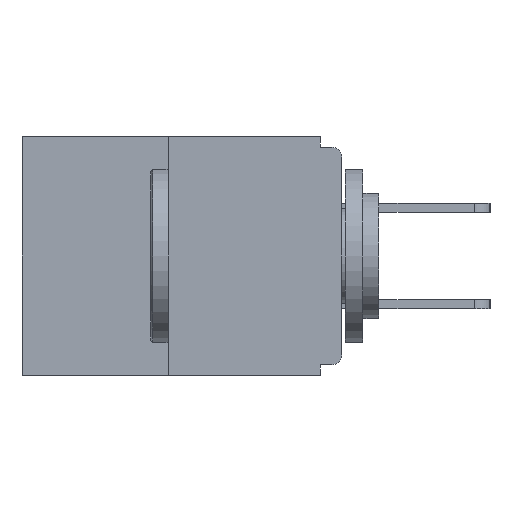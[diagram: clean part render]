
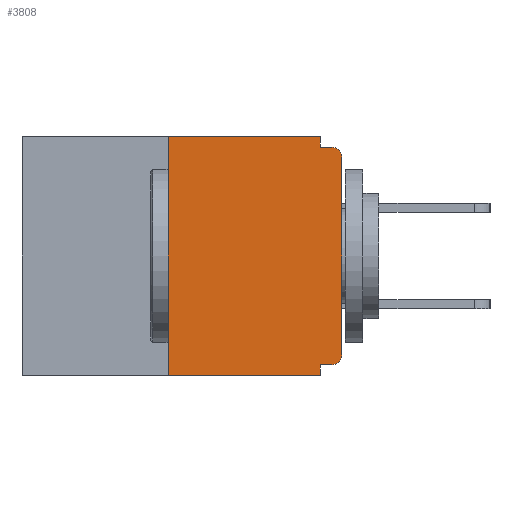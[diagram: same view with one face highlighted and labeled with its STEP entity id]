
A CAD part, left-side view. The second image highlights one B-rep face of the part: STEP entity #3808.
In plain terms, the highlighted planar face has unit normal (-1, 0, 0).
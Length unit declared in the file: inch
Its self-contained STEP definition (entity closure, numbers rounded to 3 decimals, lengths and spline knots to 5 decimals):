
#72 = LINE ( 'NONE', #8200, #8737 ) ;
#194 = CARTESIAN_POINT ( 'NONE',  ( 0., 0.031, -0.328 ) ) ;
#492 = LINE ( 'NONE', #3916, #2522 ) ;
#623 = LINE ( 'NONE', #11089, #8956 ) ;
#651 = ORIENTED_EDGE ( 'NONE', *, *, #4061, .T. ) ;
#663 = CARTESIAN_POINT ( 'NONE',  ( 0., 0.015, -0.328 ) ) ;
#784 = VECTOR ( 'NONE', #2452, 39.37008 ) ;
#804 = VERTEX_POINT ( 'NONE', #7273 ) ;
#844 = DIRECTION ( 'NONE',  ( -1., 0., 0. ) ) ;
#850 = DIRECTION ( 'NONE',  ( 0., 0., -1. ) ) ;
#1008 = AXIS2_PLACEMENT_3D ( 'NONE', #3945, #1870, #2927 ) ;
#1231 = EDGE_CURVE ( 'NONE', #7471, #804, #9520, .T. ) ;
#1250 = CARTESIAN_POINT ( 'NONE',  ( 0., 0.015, -0.015 ) ) ;
#1302 = ORIENTED_EDGE ( 'NONE', *, *, #5220, .F. ) ;
#1521 = EDGE_CURVE ( 'NONE', #3811, #3905, #72, .T. ) ;
#1755 = VERTEX_POINT ( 'NONE', #3054 ) ;
#1815 = CARTESIAN_POINT ( 'NONE',  ( 0., 0.031, -0.343 ) ) ;
#1870 = DIRECTION ( 'NONE',  ( -1., 0., 0. ) ) ;
#1968 = DIRECTION ( 'NONE',  ( 0., 0., -1. ) ) ;
#1997 = DIRECTION ( 'NONE',  ( 0., -1., 0. ) ) ;
#2021 = LINE ( 'NONE', #8371, #784 ) ;
#2122 = ORIENTED_EDGE ( 'NONE', *, *, #1521, .F. ) ;
#2430 = CARTESIAN_POINT ( 'NONE',  ( 0., 0.46, 0. ) ) ;
#2452 = DIRECTION ( 'NONE',  ( 0., 0., 1. ) ) ;
#2522 = VECTOR ( 'NONE', #11667, 39.37008 ) ;
#2750 = CARTESIAN_POINT ( 'NONE',  ( 0., 0.031, 0. ) ) ;
#2927 = DIRECTION ( 'NONE',  ( 0., 0., -1. ) ) ;
#2958 = LINE ( 'NONE', #2750, #9585 ) ;
#3054 = CARTESIAN_POINT ( 'NONE',  ( 0., 0.031, -0.015 ) ) ;
#3327 = DIRECTION ( 'NONE',  ( 0., 0., -1. ) ) ;
#3495 = PLANE ( 'NONE',  #10316 ) ;
#3754 = VERTEX_POINT ( 'NONE', #194 ) ;
#3802 = VERTEX_POINT ( 'NONE', #11382 ) ;
#3808 = ADVANCED_FACE ( 'NONE', ( #6833 ), #3495, .F. ) ;
#3811 = VERTEX_POINT ( 'NONE', #6304 ) ;
#3905 = VERTEX_POINT ( 'NONE', #7506 ) ;
#3916 = CARTESIAN_POINT ( 'NONE',  ( 0., 0., -0.328 ) ) ;
#3945 = CARTESIAN_POINT ( 'NONE',  ( 0., 0.015, -0.03 ) ) ;
#4061 = EDGE_CURVE ( 'NONE', #804, #8149, #8849, .T. ) ;
#4160 = EDGE_CURVE ( 'NONE', #7471, #3754, #492, .T. ) ;
#4607 = LINE ( 'NONE', #9887, #12474 ) ;
#4749 = ORIENTED_EDGE ( 'NONE', *, *, #4160, .F. ) ;
#4822 = DIRECTION ( 'NONE',  ( 0., 0., 1. ) ) ;
#5002 = EDGE_CURVE ( 'NONE', #10737, #3811, #2021, .T. ) ;
#5121 = ORIENTED_EDGE ( 'NONE', *, *, #11349, .F. ) ;
#5173 = ORIENTED_EDGE ( 'NONE', *, *, #10249, .F. ) ;
#5220 = EDGE_CURVE ( 'NONE', #3905, #1755, #2958, .T. ) ;
#5342 = ORIENTED_EDGE ( 'NONE', *, *, #7590, .T. ) ;
#5391 = EDGE_CURVE ( 'NONE', #10737, #3802, #623, .T. ) ;
#5588 = DIRECTION ( 'NONE',  ( 0., 0., -1. ) ) ;
#5977 = VECTOR ( 'NONE', #850, 39.37008 ) ;
#6135 = DIRECTION ( 'NONE',  ( 0., -1., 0. ) ) ;
#6304 = CARTESIAN_POINT ( 'NONE',  ( 0., 0.25, 0. ) ) ;
#6742 = LINE ( 'NONE', #1815, #5977 ) ;
#6798 = CARTESIAN_POINT ( 'NONE',  ( 0., 0.015, -0.313 ) ) ;
#6833 = FACE_OUTER_BOUND ( 'NONE', #10438, .T. ) ;
#7273 = CARTESIAN_POINT ( 'NONE',  ( 0., 0., -0.313 ) ) ;
#7323 = DIRECTION ( 'NONE',  ( 1., 0., 0. ) ) ;
#7471 = VERTEX_POINT ( 'NONE', #663 ) ;
#7506 = CARTESIAN_POINT ( 'NONE',  ( 0., 0.031, 0. ) ) ;
#7590 = EDGE_CURVE ( 'NONE', #8149, #12725, #12071, .T. ) ;
#8149 = VERTEX_POINT ( 'NONE', #10561 ) ;
#8200 = CARTESIAN_POINT ( 'NONE',  ( 0., 0.46, 0. ) ) ;
#8371 = CARTESIAN_POINT ( 'NONE',  ( 0., 0.25, 0. ) ) ;
#8687 = VECTOR ( 'NONE', #4822, 39.37008 ) ;
#8737 = VECTOR ( 'NONE', #10193, 39.37008 ) ;
#8849 = LINE ( 'NONE', #12632, #8687 ) ;
#8925 = ORIENTED_EDGE ( 'NONE', *, *, #5391, .T. ) ;
#8956 = VECTOR ( 'NONE', #6135, 39.37008 ) ;
#9520 = CIRCLE ( 'NONE', #9808, 0.015 ) ;
#9585 = VECTOR ( 'NONE', #5588, 39.37008 ) ;
#9717 = CARTESIAN_POINT ( 'NONE',  ( 0., 0.25, -0.343 ) ) ;
#9808 = AXIS2_PLACEMENT_3D ( 'NONE', #6798, #844, #1968 ) ;
#9887 = CARTESIAN_POINT ( 'NONE',  ( 0., 0., -0.015 ) ) ;
#10193 = DIRECTION ( 'NONE',  ( 0., -1., 0. ) ) ;
#10249 = EDGE_CURVE ( 'NONE', #1755, #12725, #4607, .T. ) ;
#10316 = AXIS2_PLACEMENT_3D ( 'NONE', #2430, #7323, #3327 ) ;
#10438 = EDGE_LOOP ( 'NONE', ( #2122, #11658, #8925, #5121, #4749, #11987, #651, #5342, #5173, #1302 ) ) ;
#10561 = CARTESIAN_POINT ( 'NONE',  ( 0., 0., -0.03 ) ) ;
#10737 = VERTEX_POINT ( 'NONE', #9717 ) ;
#11089 = CARTESIAN_POINT ( 'NONE',  ( 0., 0.46, -0.343 ) ) ;
#11349 = EDGE_CURVE ( 'NONE', #3754, #3802, #6742, .T. ) ;
#11382 = CARTESIAN_POINT ( 'NONE',  ( 0., 0.031, -0.343 ) ) ;
#11658 = ORIENTED_EDGE ( 'NONE', *, *, #5002, .F. ) ;
#11667 = DIRECTION ( 'NONE',  ( 0., 1., 0. ) ) ;
#11987 = ORIENTED_EDGE ( 'NONE', *, *, #1231, .T. ) ;
#12071 = CIRCLE ( 'NONE', #1008, 0.015 ) ;
#12474 = VECTOR ( 'NONE', #1997, 39.37008 ) ;
#12632 = CARTESIAN_POINT ( 'NONE',  ( 0., 0., 0. ) ) ;
#12725 = VERTEX_POINT ( 'NONE', #1250 ) ;
